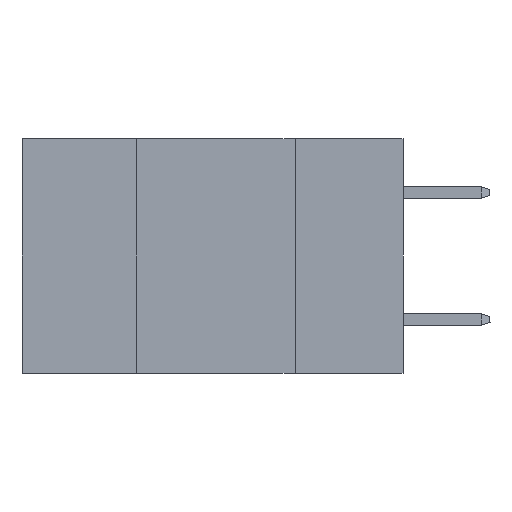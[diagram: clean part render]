
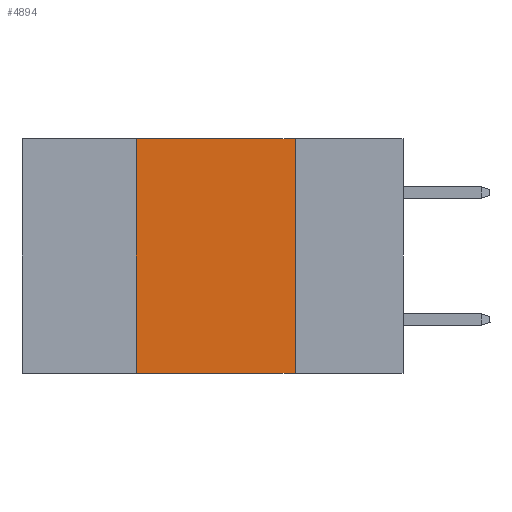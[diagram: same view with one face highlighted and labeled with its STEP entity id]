
A CAD part, left-side view. The second image highlights one B-rep face of the part: STEP entity #4894.
In plain terms, the highlighted planar face has unit normal (-1, 0, 0).
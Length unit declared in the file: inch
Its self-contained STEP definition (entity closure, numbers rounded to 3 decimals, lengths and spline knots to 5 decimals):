
#37 = AXIS2_PLACEMENT_3D ( 'NONE', #14633, #16009, #14815 ) ;
#151 = VERTEX_POINT ( 'NONE', #13964 ) ;
#788 = FACE_OUTER_BOUND ( 'NONE', #17064, .T. ) ;
#1021 = ORIENTED_EDGE ( 'NONE', *, *, #9642, .F. ) ;
#1983 = DIRECTION ( 'NONE',  ( 0., -1., 0. ) ) ;
#2690 = DIRECTION ( 'NONE',  ( 0., -1., 0. ) ) ;
#3098 = VECTOR ( 'NONE', #15811, 39.37008 ) ;
#3355 = CARTESIAN_POINT ( 'NONE',  ( 0., 0.6, -0.37 ) ) ;
#3610 = ORIENTED_EDGE ( 'NONE', *, *, #13953, .F. ) ;
#4894 = ADVANCED_FACE ( 'NONE', ( #788 ), #6474, .F. ) ;
#4988 = VECTOR ( 'NONE', #10274, 39.37008 ) ;
#5762 = CARTESIAN_POINT ( 'NONE',  ( 0., 0.17, -0.37 ) ) ;
#6221 = VECTOR ( 'NONE', #1983, 39.37008 ) ;
#6474 = PLANE ( 'NONE',  #37 ) ;
#7558 = CARTESIAN_POINT ( 'NONE',  ( 0., 0.42, 0. ) ) ;
#7577 = LINE ( 'NONE', #3355, #6221 ) ;
#7618 = VERTEX_POINT ( 'NONE', #5762 ) ;
#8885 = LINE ( 'NONE', #13023, #4988 ) ;
#8910 = ORIENTED_EDGE ( 'NONE', *, *, #17467, .F. ) ;
#9642 = EDGE_CURVE ( 'NONE', #10710, #7618, #8885, .T. ) ;
#10274 = DIRECTION ( 'NONE',  ( 0., 0., -1. ) ) ;
#10433 = VECTOR ( 'NONE', #2690, 39.37008 ) ;
#10678 = EDGE_CURVE ( 'NONE', #151, #7618, #7577, .T. ) ;
#10710 = VERTEX_POINT ( 'NONE', #12350 ) ;
#12350 = CARTESIAN_POINT ( 'NONE',  ( 0., 0.17, 0. ) ) ;
#12596 = LINE ( 'NONE', #15259, #10433 ) ;
#13023 = CARTESIAN_POINT ( 'NONE',  ( 0., 0.17, 0. ) ) ;
#13047 = LINE ( 'NONE', #17189, #3098 ) ;
#13953 = EDGE_CURVE ( 'NONE', #151, #15168, #13047, .T. ) ;
#13964 = CARTESIAN_POINT ( 'NONE',  ( 0., 0.42, -0.37 ) ) ;
#14633 = CARTESIAN_POINT ( 'NONE',  ( 0., 0.6, 0. ) ) ;
#14815 = DIRECTION ( 'NONE',  ( 0., 0., -1. ) ) ;
#15168 = VERTEX_POINT ( 'NONE', #7558 ) ;
#15259 = CARTESIAN_POINT ( 'NONE',  ( 0., 0.6, 0. ) ) ;
#15811 = DIRECTION ( 'NONE',  ( 0., 0., 1. ) ) ;
#16009 = DIRECTION ( 'NONE',  ( 1., 0., 0. ) ) ;
#16914 = ORIENTED_EDGE ( 'NONE', *, *, #10678, .T. ) ;
#17064 = EDGE_LOOP ( 'NONE', ( #1021, #8910, #3610, #16914 ) ) ;
#17189 = CARTESIAN_POINT ( 'NONE',  ( 0., 0.42, 0. ) ) ;
#17467 = EDGE_CURVE ( 'NONE', #15168, #10710, #12596, .T. ) ;
